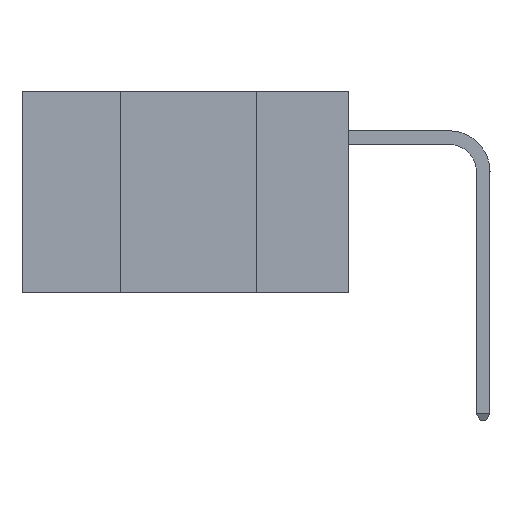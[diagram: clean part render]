
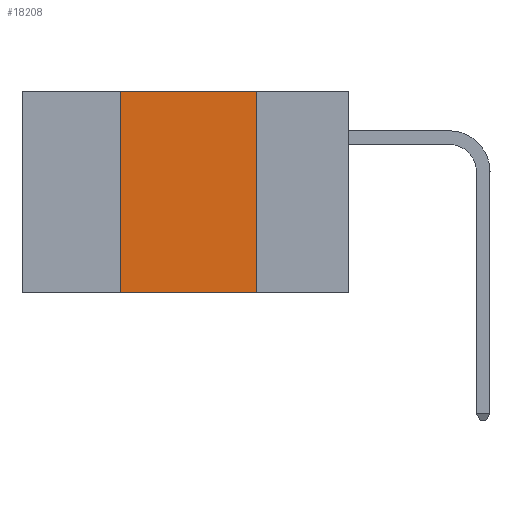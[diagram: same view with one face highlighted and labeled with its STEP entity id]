
A CAD part, left-side view. The second image highlights one B-rep face of the part: STEP entity #18208.
In plain terms, the highlighted planar face has unit normal (-1, 0, 0).
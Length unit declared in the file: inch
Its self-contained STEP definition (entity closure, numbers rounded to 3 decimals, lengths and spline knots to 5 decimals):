
#297 = VECTOR ( 'NONE', #5498, 39.37008 ) ;
#321 = VECTOR ( 'NONE', #9142, 39.37008 ) ;
#1667 = CARTESIAN_POINT ( 'NONE',  ( 0., 0.6, 0. ) ) ;
#2876 = EDGE_CURVE ( 'NONE', #10789, #11455, #13973, .T. ) ;
#3736 = CARTESIAN_POINT ( 'NONE',  ( 0., 0.6, -0.37 ) ) ;
#3809 = ORIENTED_EDGE ( 'NONE', *, *, #2876, .F. ) ;
#4164 = ORIENTED_EDGE ( 'NONE', *, *, #20398, .F. ) ;
#4220 = ORIENTED_EDGE ( 'NONE', *, *, #21308, .F. ) ;
#4324 = ORIENTED_EDGE ( 'NONE', *, *, #14705, .T. ) ;
#5019 = AXIS2_PLACEMENT_3D ( 'NONE', #9518, #9591, #21188 ) ;
#5137 = DIRECTION ( 'NONE',  ( 0., -1., 0. ) ) ;
#5173 = LINE ( 'NONE', #3736, #297 ) ;
#5259 = LINE ( 'NONE', #1667, #9292 ) ;
#5498 = DIRECTION ( 'NONE',  ( 0., -1., 0. ) ) ;
#6474 = CARTESIAN_POINT ( 'NONE',  ( 0., 0.17, 0. ) ) ;
#8342 = VERTEX_POINT ( 'NONE', #20253 ) ;
#9142 = DIRECTION ( 'NONE',  ( 0., 0., -1. ) ) ;
#9292 = VECTOR ( 'NONE', #5137, 39.37008 ) ;
#9518 = CARTESIAN_POINT ( 'NONE',  ( 0., 0.6, 0. ) ) ;
#9591 = DIRECTION ( 'NONE',  ( 1., 0., 0. ) ) ;
#10789 = VERTEX_POINT ( 'NONE', #6474 ) ;
#11084 = CARTESIAN_POINT ( 'NONE',  ( 0., 0.42, 0. ) ) ;
#11455 = VERTEX_POINT ( 'NONE', #16201 ) ;
#12526 = FACE_OUTER_BOUND ( 'NONE', #14504, .T. ) ;
#12732 = DIRECTION ( 'NONE',  ( 0., 0., 1. ) ) ;
#13463 = LINE ( 'NONE', #11084, #16881 ) ;
#13973 = LINE ( 'NONE', #17487, #321 ) ;
#14504 = EDGE_LOOP ( 'NONE', ( #3809, #4164, #4220, #4324 ) ) ;
#14705 = EDGE_CURVE ( 'NONE', #15854, #11455, #5173, .T. ) ;
#15854 = VERTEX_POINT ( 'NONE', #16897 ) ;
#16201 = CARTESIAN_POINT ( 'NONE',  ( 0., 0.17, -0.37 ) ) ;
#16249 = PLANE ( 'NONE',  #5019 ) ;
#16881 = VECTOR ( 'NONE', #12732, 39.37008 ) ;
#16897 = CARTESIAN_POINT ( 'NONE',  ( 0., 0.42, -0.37 ) ) ;
#17487 = CARTESIAN_POINT ( 'NONE',  ( 0., 0.17, 0. ) ) ;
#18208 = ADVANCED_FACE ( 'NONE', ( #12526 ), #16249, .F. ) ;
#20253 = CARTESIAN_POINT ( 'NONE',  ( 0., 0.42, 0. ) ) ;
#20398 = EDGE_CURVE ( 'NONE', #8342, #10789, #5259, .T. ) ;
#21188 = DIRECTION ( 'NONE',  ( 0., 0., -1. ) ) ;
#21308 = EDGE_CURVE ( 'NONE', #15854, #8342, #13463, .T. ) ;
